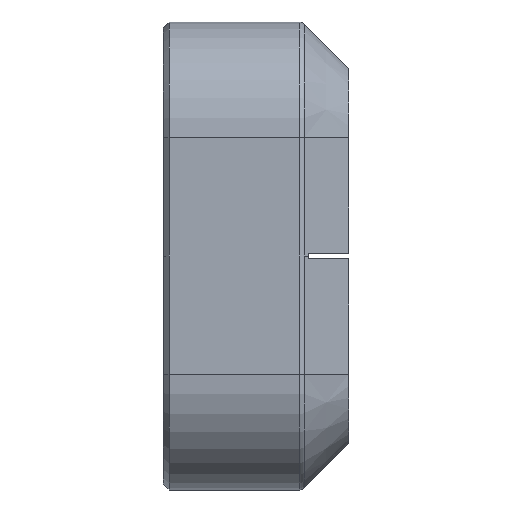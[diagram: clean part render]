
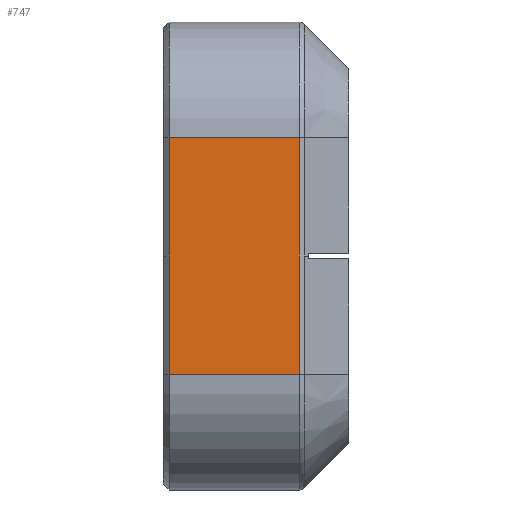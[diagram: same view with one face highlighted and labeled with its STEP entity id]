
A CAD part, left-side view. The second image highlights one B-rep face of the part: STEP entity #747.
In plain terms, the highlighted planar face has unit normal (-1, 0, 0).
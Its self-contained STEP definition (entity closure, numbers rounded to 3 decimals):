
#46 = EDGE_CURVE ( 'NONE', #6014, #8250, #186, .T. ) ;
#186 = LINE ( 'NONE', #4065, #7146 ) ;
#489 = EDGE_CURVE ( 'NONE', #3955, #4647, #4851, .T. ) ;
#747 = ADVANCED_FACE ( 'NONE', ( #2681 ), #3347, .F. ) ;
#1167 = AXIS2_PLACEMENT_3D ( 'NONE', #5772, #4471, #5220 ) ;
#1486 = LINE ( 'NONE', #5358, #4097 ) ;
#1530 = EDGE_CURVE ( 'NONE', #4647, #6014, #3360, .T. ) ;
#1568 = VECTOR ( 'NONE', #5151, 1000. ) ;
#1988 = DIRECTION ( 'NONE',  ( 0., -1., 0. ) ) ;
#2020 = EDGE_LOOP ( 'NONE', ( #2434, #6184, #7229, #7289 ) ) ;
#2195 = CARTESIAN_POINT ( 'NONE',  ( -34., -10.2, 10. ) ) ;
#2356 = CARTESIAN_POINT ( 'NONE',  ( -34., 10.2, -5.5 ) ) ;
#2434 = ORIENTED_EDGE ( 'NONE', *, *, #489, .T. ) ;
#2681 = FACE_OUTER_BOUND ( 'NONE', #2020, .T. ) ;
#3347 = PLANE ( 'NONE',  #1167 ) ;
#3360 = LINE ( 'NONE', #4533, #1568 ) ;
#3955 = VERTEX_POINT ( 'NONE', #8137 ) ;
#4065 = CARTESIAN_POINT ( 'NONE',  ( -34., 10.2, 5. ) ) ;
#4097 = VECTOR ( 'NONE', #1988, 1000. ) ;
#4471 = DIRECTION ( 'NONE',  ( 1., 0., 0. ) ) ;
#4533 = CARTESIAN_POINT ( 'NONE',  ( -34., 10.2, 5.751 ) ) ;
#4647 = VERTEX_POINT ( 'NONE', #8059 ) ;
#4851 = LINE ( 'NONE', #2195, #6218 ) ;
#5151 = DIRECTION ( 'NONE',  ( 0., 1., 0. ) ) ;
#5220 = DIRECTION ( 'NONE',  ( 0., 1., 0. ) ) ;
#5358 = CARTESIAN_POINT ( 'NONE',  ( -34., -10.2, -5.5 ) ) ;
#5388 = CARTESIAN_POINT ( 'NONE',  ( -34., 10.2, 5.751 ) ) ;
#5547 = EDGE_CURVE ( 'NONE', #8250, #3955, #1486, .T. ) ;
#5772 = CARTESIAN_POINT ( 'NONE',  ( -34., 0., 5. ) ) ;
#6014 = VERTEX_POINT ( 'NONE', #5388 ) ;
#6184 = ORIENTED_EDGE ( 'NONE', *, *, #1530, .T. ) ;
#6218 = VECTOR ( 'NONE', #8031, 1000. ) ;
#7146 = VECTOR ( 'NONE', #7319, 1000. ) ;
#7229 = ORIENTED_EDGE ( 'NONE', *, *, #46, .T. ) ;
#7289 = ORIENTED_EDGE ( 'NONE', *, *, #5547, .T. ) ;
#7319 = DIRECTION ( 'NONE',  ( 0., 0., -1. ) ) ;
#8031 = DIRECTION ( 'NONE',  ( 0., 0., 1. ) ) ;
#8059 = CARTESIAN_POINT ( 'NONE',  ( -34., -10.2, 5.751 ) ) ;
#8137 = CARTESIAN_POINT ( 'NONE',  ( -34., -10.2, -5.5 ) ) ;
#8250 = VERTEX_POINT ( 'NONE', #2356 ) ;
